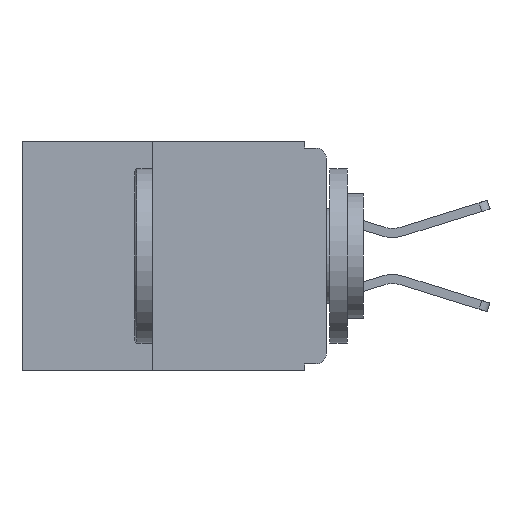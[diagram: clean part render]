
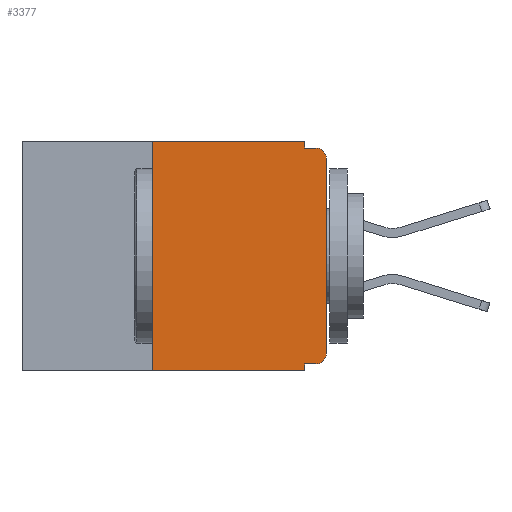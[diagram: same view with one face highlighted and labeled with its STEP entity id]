
A CAD part, left-side view. The second image highlights one B-rep face of the part: STEP entity #3377.
In plain terms, the highlighted planar face has unit normal (-1, 0, 0).
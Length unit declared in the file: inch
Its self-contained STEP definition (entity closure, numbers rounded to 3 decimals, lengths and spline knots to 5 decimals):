
#4 = DIRECTION ( 'NONE',  ( 0., 0., -1. ) ) ;
#667 = CARTESIAN_POINT ( 'NONE',  ( 0., 0., 0. ) ) ;
#741 = VERTEX_POINT ( 'NONE', #24903 ) ;
#1644 = VECTOR ( 'NONE', #4, 39.37008 ) ;
#1716 = CARTESIAN_POINT ( 'NONE',  ( 0., 0., -0.025 ) ) ;
#1734 = EDGE_CURVE ( 'NONE', #6913, #17517, #15999, .T. ) ;
#1782 = DIRECTION ( 'NONE',  ( 0., 0., -1. ) ) ;
#1789 = DIRECTION ( 'NONE',  ( 1., 0., 0. ) ) ;
#1885 = VERTEX_POINT ( 'NONE', #1716 ) ;
#1961 = CARTESIAN_POINT ( 'NONE',  ( 0., 0.437, 0. ) ) ;
#2234 = CARTESIAN_POINT ( 'NONE',  ( 0., 0.031, 0. ) ) ;
#2777 = CARTESIAN_POINT ( 'NONE',  ( 0., 0.25, -0.33 ) ) ;
#3198 = PLANE ( 'NONE',  #15565 ) ;
#3377 = ADVANCED_FACE ( 'NONE', ( #25369 ), #3198, .F. ) ;
#3669 = ORIENTED_EDGE ( 'NONE', *, *, #12428, .T. ) ;
#3796 = CARTESIAN_POINT ( 'NONE',  ( 0., 0., -0.01 ) ) ;
#3867 = VECTOR ( 'NONE', #4111, 39.37008 ) ;
#3930 = ORIENTED_EDGE ( 'NONE', *, *, #8743, .T. ) ;
#4111 = DIRECTION ( 'NONE',  ( 0., 0., -1. ) ) ;
#4312 = CARTESIAN_POINT ( 'NONE',  ( 0., 0.25, 0. ) ) ;
#4508 = VECTOR ( 'NONE', #25798, 39.37008 ) ;
#4826 = VECTOR ( 'NONE', #26388, 39.37008 ) ;
#4894 = ORIENTED_EDGE ( 'NONE', *, *, #24095, .F. ) ;
#5349 = ORIENTED_EDGE ( 'NONE', *, *, #10498, .F. ) ;
#5886 = ORIENTED_EDGE ( 'NONE', *, *, #1734, .F. ) ;
#5897 = LINE ( 'NONE', #11266, #4508 ) ;
#5914 = EDGE_CURVE ( 'NONE', #26429, #6248, #17445, .T. ) ;
#6047 = VERTEX_POINT ( 'NONE', #2777 ) ;
#6122 = VECTOR ( 'NONE', #25557, 39.37008 ) ;
#6248 = VERTEX_POINT ( 'NONE', #23120 ) ;
#6330 = CARTESIAN_POINT ( 'NONE',  ( 0., 0.031, -0.33 ) ) ;
#6334 = ORIENTED_EDGE ( 'NONE', *, *, #9083, .F. ) ;
#6419 = ORIENTED_EDGE ( 'NONE', *, *, #15176, .T. ) ;
#6578 = ORIENTED_EDGE ( 'NONE', *, *, #8179, .F. ) ;
#6614 = ORIENTED_EDGE ( 'NONE', *, *, #14318, .F. ) ;
#6795 = ORIENTED_EDGE ( 'NONE', *, *, #5914, .T. ) ;
#6913 = VERTEX_POINT ( 'NONE', #4312 ) ;
#6918 = CIRCLE ( 'NONE', #10966, 0.015 ) ;
#7346 = CARTESIAN_POINT ( 'NONE',  ( 0., 0.031, -0.01 ) ) ;
#7715 = LINE ( 'NONE', #3796, #18750 ) ;
#8075 = CARTESIAN_POINT ( 'NONE',  ( 0., 0.437, 0. ) ) ;
#8179 = EDGE_CURVE ( 'NONE', #11139, #741, #20656, .T. ) ;
#8743 = EDGE_CURVE ( 'NONE', #1885, #16502, #6918, .T. ) ;
#8783 = LINE ( 'NONE', #2234, #1644 ) ;
#9083 = EDGE_CURVE ( 'NONE', #6047, #6913, #5897, .T. ) ;
#9970 = CARTESIAN_POINT ( 'NONE',  ( 0., 0., -0.32 ) ) ;
#10187 = DIRECTION ( 'NONE',  ( -1., 0., 0. ) ) ;
#10414 = LINE ( 'NONE', #11033, #6122 ) ;
#10498 = EDGE_CURVE ( 'NONE', #17517, #26293, #8783, .T. ) ;
#10966 = AXIS2_PLACEMENT_3D ( 'NONE', #22625, #10187, #24705 ) ;
#11033 = CARTESIAN_POINT ( 'NONE',  ( 0., 0.437, -0.33 ) ) ;
#11139 = VERTEX_POINT ( 'NONE', #23180 ) ;
#11266 = CARTESIAN_POINT ( 'NONE',  ( 0., 0.25, -0.33 ) ) ;
#12428 = EDGE_CURVE ( 'NONE', #6248, #1885, #15090, .T. ) ;
#12811 = AXIS2_PLACEMENT_3D ( 'NONE', #14704, #14666, #13893 ) ;
#13485 = DIRECTION ( 'NONE',  ( 0., 0., 1. ) ) ;
#13893 = DIRECTION ( 'NONE',  ( 0., 0., -1. ) ) ;
#14318 = EDGE_CURVE ( 'NONE', #26429, #11139, #14662, .T. ) ;
#14422 = VECTOR ( 'NONE', #13485, 39.37008 ) ;
#14662 = LINE ( 'NONE', #9970, #26369 ) ;
#14666 = DIRECTION ( 'NONE',  ( -1., 0., 0. ) ) ;
#14704 = CARTESIAN_POINT ( 'NONE',  ( 0., 0.015, -0.305 ) ) ;
#15090 = LINE ( 'NONE', #667, #14422 ) ;
#15176 = EDGE_CURVE ( 'NONE', #6047, #741, #10414, .T. ) ;
#15565 = AXIS2_PLACEMENT_3D ( 'NONE', #1961, #1789, #1782 ) ;
#15999 = LINE ( 'NONE', #8075, #4826 ) ;
#16414 = DIRECTION ( 'NONE',  ( 0., -1., 0. ) ) ;
#16502 = VERTEX_POINT ( 'NONE', #24796 ) ;
#17445 = CIRCLE ( 'NONE', #12811, 0.015 ) ;
#17517 = VERTEX_POINT ( 'NONE', #24034 ) ;
#18750 = VECTOR ( 'NONE', #16414, 39.37008 ) ;
#20598 = EDGE_LOOP ( 'NONE', ( #3669, #3930, #4894, #5349, #5886, #6334, #6419, #6578, #6614, #6795 ) ) ;
#20656 = LINE ( 'NONE', #6330, #3867 ) ;
#22625 = CARTESIAN_POINT ( 'NONE',  ( 0., 0.015, -0.025 ) ) ;
#23120 = CARTESIAN_POINT ( 'NONE',  ( 0., 0., -0.305 ) ) ;
#23180 = CARTESIAN_POINT ( 'NONE',  ( 0., 0.031, -0.32 ) ) ;
#24034 = CARTESIAN_POINT ( 'NONE',  ( 0., 0.031, 0. ) ) ;
#24095 = EDGE_CURVE ( 'NONE', #26293, #16502, #7715, .T. ) ;
#24436 = CARTESIAN_POINT ( 'NONE',  ( 0., 0.015, -0.32 ) ) ;
#24483 = DIRECTION ( 'NONE',  ( 0., 1., 0. ) ) ;
#24705 = DIRECTION ( 'NONE',  ( 0., 0., -1. ) ) ;
#24796 = CARTESIAN_POINT ( 'NONE',  ( 0., 0.015, -0.01 ) ) ;
#24903 = CARTESIAN_POINT ( 'NONE',  ( 0., 0.031, -0.33 ) ) ;
#25369 = FACE_OUTER_BOUND ( 'NONE', #20598, .T. ) ;
#25557 = DIRECTION ( 'NONE',  ( 0., -1., 0. ) ) ;
#25798 = DIRECTION ( 'NONE',  ( 0., 0., 1. ) ) ;
#26293 = VERTEX_POINT ( 'NONE', #7346 ) ;
#26369 = VECTOR ( 'NONE', #24483, 39.37008 ) ;
#26388 = DIRECTION ( 'NONE',  ( 0., -1., 0. ) ) ;
#26429 = VERTEX_POINT ( 'NONE', #24436 ) ;
